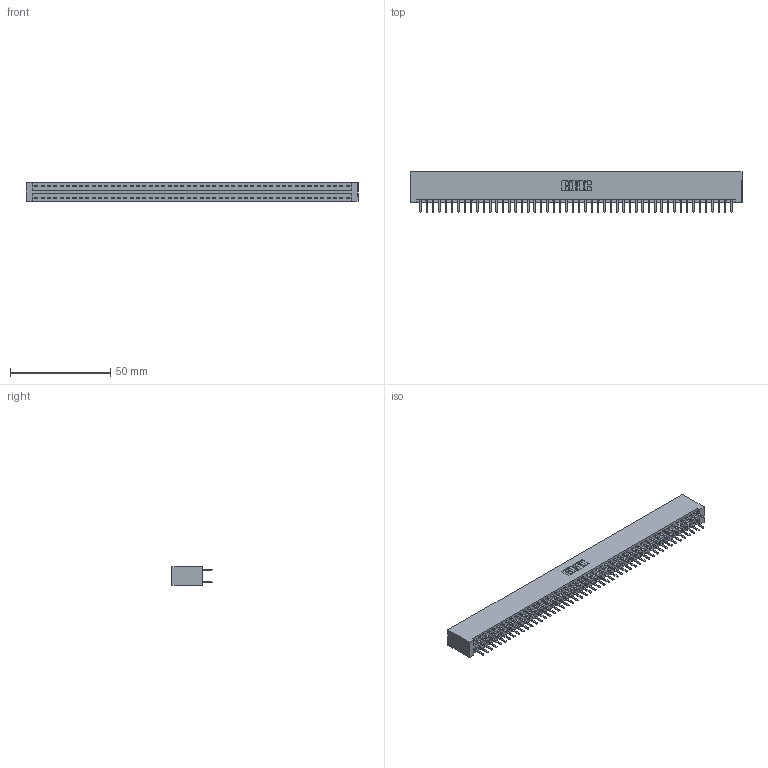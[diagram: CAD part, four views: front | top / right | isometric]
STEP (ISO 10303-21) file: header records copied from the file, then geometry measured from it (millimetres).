
FILE_DESCRIPTION (( 'STEP AP203' ), '1' );
FILE_NAME ('396-100-520-201.STEP', '2018-09-14T06:23:09', ( '' ), ( '' ), 'SwSTEP 2.0', 'SolidWorks 2016', '' );
FILE_SCHEMA (( 'CONFIG_CONTROL_DESIGN' ));
Length unit declared in the file: inch
Products named in the file (3): 346 Part_No Mounting Lugs; 345-292-001_345-293-120; 396-100-520-201
Assembly tree (101 placements, depth 2):
  396-100-520-201
    346 Part_No Mounting Lugs
    345-292-001_345-293-120  x100
Bounding box: 165.99 x 20.02 x 9.4 mm (x, y, z)
Volume: 16777.4 mm3; surface area: 23247.7 mm2
Topology: 101 solids, 101 shells, 5714 faces, 16605 edges, 10802 vertices
Faces by surface type: plane 3772, cylinder 1942
Entity records: 31391 total; most frequent: CARTESIAN_POINT 5172, ORIENTED_EDGE 5094, DIRECTION 4591, EDGE_CURVE 2547, LINE 2219, VECTOR 2219, VERTEX_POINT 1694, AXIS2_PLACEMENT_3D 1186
